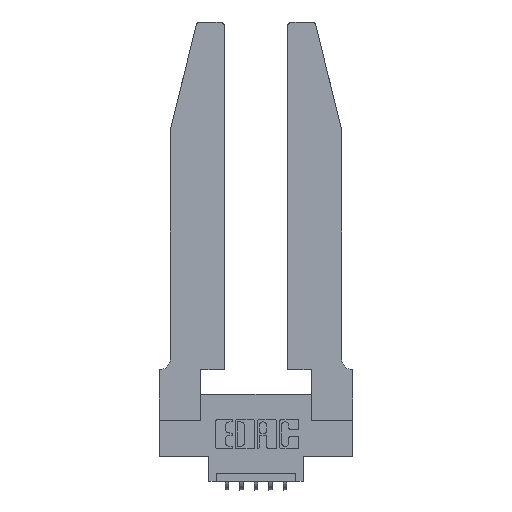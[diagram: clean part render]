
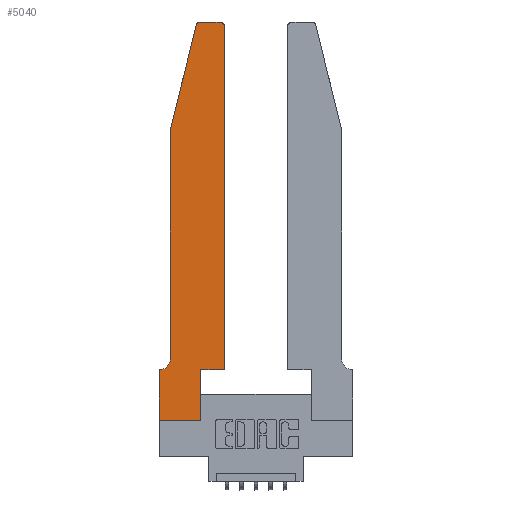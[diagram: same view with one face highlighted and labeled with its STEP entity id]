
A CAD part, top view. The second image highlights one B-rep face of the part: STEP entity #5040.
In plain terms, the highlighted planar face has unit normal (0, 0, 1).
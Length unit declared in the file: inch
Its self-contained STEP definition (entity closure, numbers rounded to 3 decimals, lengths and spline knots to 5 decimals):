
#56 = CARTESIAN_POINT ( 'NONE',  ( 0.2865, 0.35, 0.37 ) ) ;
#78 = VERTEX_POINT ( 'NONE', #4756 ) ;
#269 = ORIENTED_EDGE ( 'NONE', *, *, #11643, .T. ) ;
#422 = CARTESIAN_POINT ( 'NONE',  ( 0.0755, 2., 0.37 ) ) ;
#649 = ORIENTED_EDGE ( 'NONE', *, *, #1210, .T. ) ;
#866 = VERTEX_POINT ( 'NONE', #9313 ) ;
#900 = DIRECTION ( 'NONE',  ( 1., 0., 0. ) ) ;
#1210 = EDGE_CURVE ( 'NONE', #866, #5206, #12834, .T. ) ;
#1276 = DIRECTION ( 'NONE',  ( 1., 0., 0. ) ) ;
#1339 = DIRECTION ( 'NONE',  ( -1., 0., 0. ) ) ;
#1404 = VECTOR ( 'NONE', #8937, 39.37008 ) ;
#1482 = VECTOR ( 'NONE', #11932, 39.37008 ) ;
#1563 = CARTESIAN_POINT ( 'NONE',  ( 0.2605, 2.75, 0.37 ) ) ;
#1623 = EDGE_CURVE ( 'NONE', #2960, #12949, #11177, .T. ) ;
#1658 = DIRECTION ( 'NONE',  ( 1., 0., 0. ) ) ;
#1670 = ORIENTED_EDGE ( 'NONE', *, *, #11431, .T. ) ;
#1846 = LINE ( 'NONE', #11990, #7421 ) ;
#2108 = CARTESIAN_POINT ( 'NONE',  ( 0.25487, 2.72718, 0.37 ) ) ;
#2494 = CIRCLE ( 'NONE', #13128, 0.07 ) ;
#2754 = EDGE_CURVE ( 'NONE', #78, #3739, #13569, .T. ) ;
#2811 = VECTOR ( 'NONE', #13515, 39.37008 ) ;
#2960 = VERTEX_POINT ( 'NONE', #9755 ) ;
#3047 = CARTESIAN_POINT ( 'NONE',  ( 0.4205, 2.75, 0.37 ) ) ;
#3147 = ORIENTED_EDGE ( 'NONE', *, *, #4379, .T. ) ;
#3484 = PLANE ( 'NONE',  #5886 ) ;
#3739 = VERTEX_POINT ( 'NONE', #8924 ) ;
#3884 = ORIENTED_EDGE ( 'NONE', *, *, #10296, .T. ) ;
#4262 = LINE ( 'NONE', #13196, #13695 ) ;
#4294 = LINE ( 'NONE', #10812, #11248 ) ;
#4312 = VERTEX_POINT ( 'NONE', #11943 ) ;
#4379 = EDGE_CURVE ( 'NONE', #3739, #13553, #4262, .T. ) ;
#4565 = CARTESIAN_POINT ( 'NONE',  ( 0., 0.35, 0.37 ) ) ;
#4580 = CARTESIAN_POINT ( 'NONE',  ( 0.0755, 0.35, 0.37 ) ) ;
#4665 = LINE ( 'NONE', #1563, #12779 ) ;
#4756 = CARTESIAN_POINT ( 'NONE',  ( 0.2865, 0.35, 0.37 ) ) ;
#5040 = ADVANCED_FACE ( 'NONE', ( #9864 ), #3484, .T. ) ;
#5206 = VERTEX_POINT ( 'NONE', #2108 ) ;
#5312 = ORIENTED_EDGE ( 'NONE', *, *, #13296, .T. ) ;
#5518 = CARTESIAN_POINT ( 'NONE',  ( 0., 0., 0.37 ) ) ;
#5523 = ORIENTED_EDGE ( 'NONE', *, *, #8614, .T. ) ;
#5563 = DIRECTION ( 'NONE',  ( 0., 0., 1. ) ) ;
#5886 = AXIS2_PLACEMENT_3D ( 'NONE', #4565, #5563, #1276 ) ;
#6357 = DIRECTION ( 'NONE',  ( 0., 1., 0. ) ) ;
#6359 = DIRECTION ( 'NONE',  ( -1., 0., 0. ) ) ;
#6395 = LINE ( 'NONE', #56, #9359 ) ;
#6503 = ORIENTED_EDGE ( 'NONE', *, *, #10326, .T. ) ;
#6721 = VERTEX_POINT ( 'NONE', #422 ) ;
#6846 = VERTEX_POINT ( 'NONE', #3047 ) ;
#7013 = DIRECTION ( 'NONE',  ( 0., 1., 0. ) ) ;
#7018 = EDGE_LOOP ( 'NONE', ( #6503, #649, #3884, #12021, #1670, #13313, #12140, #269, #5312, #7076, #3147, #5523 ) ) ;
#7076 = ORIENTED_EDGE ( 'NONE', *, *, #2754, .T. ) ;
#7295 = CARTESIAN_POINT ( 'NONE',  ( 0.0055, 0.35, 0.37 ) ) ;
#7408 = EDGE_CURVE ( 'NONE', #12719, #2960, #8805, .T. ) ;
#7421 = VECTOR ( 'NONE', #10872, 39.37008 ) ;
#7505 = CARTESIAN_POINT ( 'NONE',  ( 0.0055, 0.42, 0.37 ) ) ;
#7882 = DIRECTION ( 'NONE',  ( -1., 0., 0. ) ) ;
#7932 = DIRECTION ( 'NONE',  ( 0., 0., 1. ) ) ;
#8266 = CARTESIAN_POINT ( 'NONE',  ( 0.284, 2.72, 0.37 ) ) ;
#8614 = EDGE_CURVE ( 'NONE', #13553, #6846, #12447, .T. ) ;
#8805 = LINE ( 'NONE', #4580, #9462 ) ;
#8869 = CARTESIAN_POINT ( 'NONE',  ( 0.4505, 2.72, 0.37 ) ) ;
#8924 = CARTESIAN_POINT ( 'NONE',  ( 0.4505, 0.35, 0.37 ) ) ;
#8937 = DIRECTION ( 'NONE',  ( 0., -1., 0. ) ) ;
#9313 = CARTESIAN_POINT ( 'NONE',  ( 0.284, 2.75, 0.37 ) ) ;
#9359 = VECTOR ( 'NONE', #6357, 39.37008 ) ;
#9366 = AXIS2_PLACEMENT_3D ( 'NONE', #8266, #9429, #900 ) ;
#9429 = DIRECTION ( 'NONE',  ( 0., 0., 1. ) ) ;
#9462 = VECTOR ( 'NONE', #1339, 39.37008 ) ;
#9627 = DIRECTION ( 'NONE',  ( 0., 0., -1. ) ) ;
#9755 = CARTESIAN_POINT ( 'NONE',  ( 0., 0.35, 0.37 ) ) ;
#9813 = DIRECTION ( 'NONE',  ( 0., -1., 0. ) ) ;
#9864 = FACE_OUTER_BOUND ( 'NONE', #7018, .T. ) ;
#10251 = LINE ( 'NONE', #5518, #1482 ) ;
#10296 = EDGE_CURVE ( 'NONE', #5206, #6721, #1846, .T. ) ;
#10326 = EDGE_CURVE ( 'NONE', #6846, #866, #4665, .T. ) ;
#10812 = CARTESIAN_POINT ( 'NONE',  ( 0.0755, 2., 0.37 ) ) ;
#10872 = DIRECTION ( 'NONE',  ( -0.239, -0.971, 0. ) ) ;
#11052 = CARTESIAN_POINT ( 'NONE',  ( 0., 0., 0.37 ) ) ;
#11177 = LINE ( 'NONE', #11052, #1404 ) ;
#11248 = VECTOR ( 'NONE', #9813, 39.37008 ) ;
#11406 = CARTESIAN_POINT ( 'NONE',  ( 0.4505, 0.35, 0.37 ) ) ;
#11431 = EDGE_CURVE ( 'NONE', #11795, #12719, #2494, .T. ) ;
#11631 = EDGE_CURVE ( 'NONE', #6721, #11795, #4294, .T. ) ;
#11643 = EDGE_CURVE ( 'NONE', #12949, #4312, #10251, .T. ) ;
#11795 = VERTEX_POINT ( 'NONE', #12150 ) ;
#11932 = DIRECTION ( 'NONE',  ( 1., 0., 0. ) ) ;
#11943 = CARTESIAN_POINT ( 'NONE',  ( 0.2865, 0., 0.37 ) ) ;
#11990 = CARTESIAN_POINT ( 'NONE',  ( 0.0755, 2., 0.37 ) ) ;
#12021 = ORIENTED_EDGE ( 'NONE', *, *, #11631, .T. ) ;
#12140 = ORIENTED_EDGE ( 'NONE', *, *, #1623, .T. ) ;
#12150 = CARTESIAN_POINT ( 'NONE',  ( 0.0755, 0.42, 0.37 ) ) ;
#12447 = CIRCLE ( 'NONE', #12930, 0.03 ) ;
#12719 = VERTEX_POINT ( 'NONE', #7295 ) ;
#12779 = VECTOR ( 'NONE', #7882, 39.37008 ) ;
#12834 = CIRCLE ( 'NONE', #9366, 0.03 ) ;
#12930 = AXIS2_PLACEMENT_3D ( 'NONE', #13246, #7932, #1658 ) ;
#12949 = VERTEX_POINT ( 'NONE', #13070 ) ;
#13070 = CARTESIAN_POINT ( 'NONE',  ( 0., 0., 0.37 ) ) ;
#13128 = AXIS2_PLACEMENT_3D ( 'NONE', #7505, #9627, #6359 ) ;
#13196 = CARTESIAN_POINT ( 'NONE',  ( 0.4505, 0.35, 0.37 ) ) ;
#13246 = CARTESIAN_POINT ( 'NONE',  ( 0.4205, 2.72, 0.37 ) ) ;
#13296 = EDGE_CURVE ( 'NONE', #4312, #78, #6395, .T. ) ;
#13313 = ORIENTED_EDGE ( 'NONE', *, *, #7408, .T. ) ;
#13515 = DIRECTION ( 'NONE',  ( 1., 0., 0. ) ) ;
#13553 = VERTEX_POINT ( 'NONE', #8869 ) ;
#13569 = LINE ( 'NONE', #11406, #2811 ) ;
#13695 = VECTOR ( 'NONE', #7013, 39.37008 ) ;
